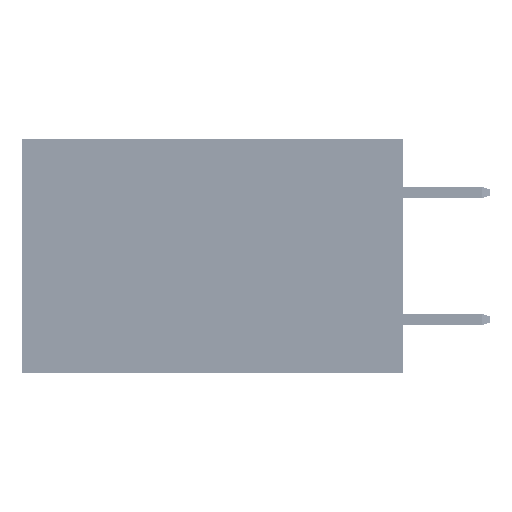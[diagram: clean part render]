
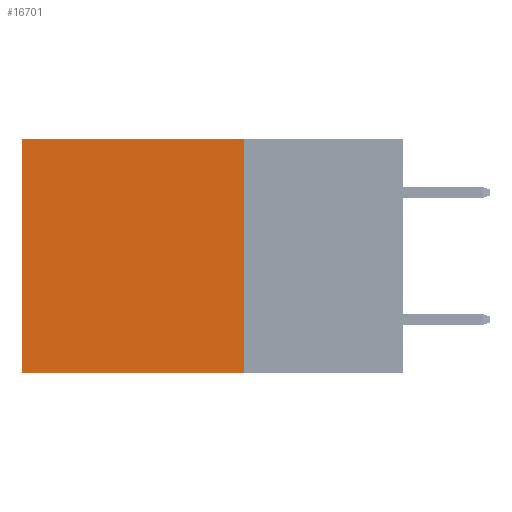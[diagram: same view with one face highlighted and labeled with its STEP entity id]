
A CAD part, left-side view. The second image highlights one B-rep face of the part: STEP entity #16701.
In plain terms, the highlighted planar face has unit normal (-1, 0, 0).
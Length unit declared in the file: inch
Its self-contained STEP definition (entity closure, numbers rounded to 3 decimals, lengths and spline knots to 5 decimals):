
#2076 = CARTESIAN_POINT ( 'NONE',  ( 0.2875, 0.25, 0. ) ) ;
#2438 = AXIS2_PLACEMENT_3D ( 'NONE', #45918, #14115, #17546 ) ;
#4125 = ORIENTED_EDGE ( 'NONE', *, *, #38820, .T. ) ;
#7270 = CARTESIAN_POINT ( 'NONE',  ( 0.2875, 0.25, 0. ) ) ;
#10372 = LINE ( 'NONE', #38747, #32915 ) ;
#14115 = DIRECTION ( 'NONE',  ( 1., 0., 0. ) ) ;
#16541 = ORIENTED_EDGE ( 'NONE', *, *, #43118, .F. ) ;
#16701 = ADVANCED_FACE ( 'NONE', ( #50127 ), #17042, .F. ) ;
#17042 = PLANE ( 'NONE',  #2438 ) ;
#17546 = DIRECTION ( 'NONE',  ( 0., 0., -1. ) ) ;
#19623 = VERTEX_POINT ( 'NONE', #42323 ) ;
#21284 = VECTOR ( 'NONE', #47470, 39.37008 ) ;
#22290 = EDGE_CURVE ( 'NONE', #36637, #19623, #10372, .T. ) ;
#23802 = VECTOR ( 'NONE', #42230, 39.37008 ) ;
#25788 = ORIENTED_EDGE ( 'NONE', *, *, #38886, .T. ) ;
#26191 = LINE ( 'NONE', #41725, #23802 ) ;
#26395 = DIRECTION ( 'NONE',  ( 0., 1., 0. ) ) ;
#30843 = CARTESIAN_POINT ( 'NONE',  ( 0.2875, 0.6, 0. ) ) ;
#32654 = DIRECTION ( 'NONE',  ( 0., 0., -1. ) ) ;
#32915 = VECTOR ( 'NONE', #26395, 39.37008 ) ;
#33371 = VERTEX_POINT ( 'NONE', #38174 ) ;
#34182 = VECTOR ( 'NONE', #32654, 39.37008 ) ;
#36637 = VERTEX_POINT ( 'NONE', #45909 ) ;
#38089 = LINE ( 'NONE', #2076, #34182 ) ;
#38174 = CARTESIAN_POINT ( 'NONE',  ( 0.2875, 0.25, 0. ) ) ;
#38747 = CARTESIAN_POINT ( 'NONE',  ( 0.2875, 0.25, -0.37 ) ) ;
#38820 = EDGE_CURVE ( 'NONE', #42873, #19623, #26191, .T. ) ;
#38886 = EDGE_CURVE ( 'NONE', #33371, #42873, #51682, .T. ) ;
#41725 = CARTESIAN_POINT ( 'NONE',  ( 0.2875, 0.6, 0. ) ) ;
#42230 = DIRECTION ( 'NONE',  ( 0., 0., -1. ) ) ;
#42323 = CARTESIAN_POINT ( 'NONE',  ( 0.2875, 0.6, -0.37 ) ) ;
#42873 = VERTEX_POINT ( 'NONE', #30843 ) ;
#43118 = EDGE_CURVE ( 'NONE', #33371, #36637, #38089, .T. ) ;
#43706 = ORIENTED_EDGE ( 'NONE', *, *, #22290, .F. ) ;
#45909 = CARTESIAN_POINT ( 'NONE',  ( 0.2875, 0.25, -0.37 ) ) ;
#45918 = CARTESIAN_POINT ( 'NONE',  ( 0.2875, 0.25, 0. ) ) ;
#47470 = DIRECTION ( 'NONE',  ( 0., 1., 0. ) ) ;
#50127 = FACE_OUTER_BOUND ( 'NONE', #50286, .T. ) ;
#50286 = EDGE_LOOP ( 'NONE', ( #4125, #43706, #16541, #25788 ) ) ;
#51682 = LINE ( 'NONE', #7270, #21284 ) ;
